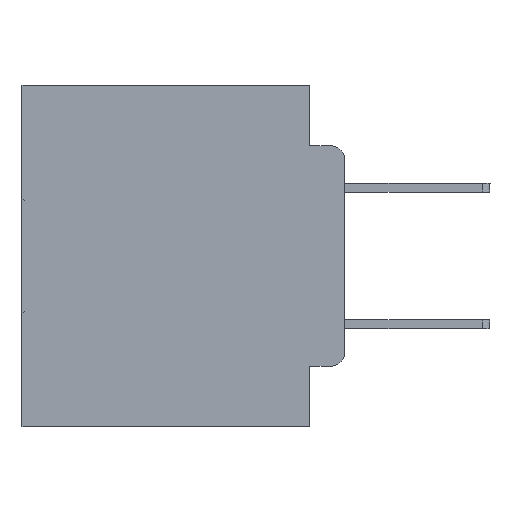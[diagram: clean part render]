
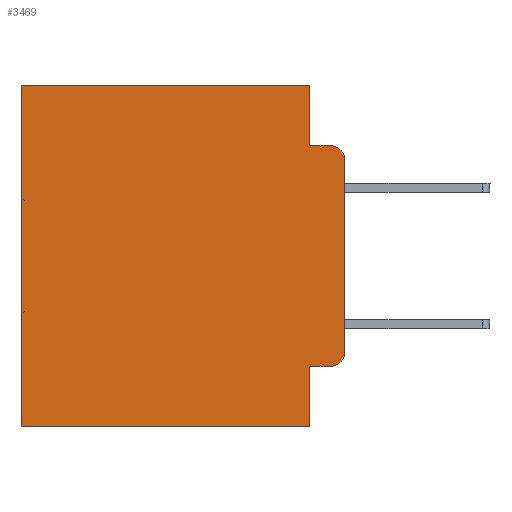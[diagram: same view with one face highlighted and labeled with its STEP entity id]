
A CAD part, left-side view. The second image highlights one B-rep face of the part: STEP entity #3469.
In plain terms, the highlighted planar face has unit normal (-1, 0, 0).
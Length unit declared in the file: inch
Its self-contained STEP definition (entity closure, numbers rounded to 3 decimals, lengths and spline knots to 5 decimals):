
#655 = PLANE ( 'NONE',  #26669 ) ;
#784 = VECTOR ( 'NONE', #4805, 39.37008 ) ;
#868 = ORIENTED_EDGE ( 'NONE', *, *, #27273, .F. ) ;
#1211 = LINE ( 'NONE', #33063, #5243 ) ;
#1711 = VERTEX_POINT ( 'NONE', #8303 ) ;
#1986 = LINE ( 'NONE', #26857, #13638 ) ;
#2028 = FACE_OUTER_BOUND ( 'NONE', #18112, .T. ) ;
#3469 = ADVANCED_FACE ( 'NONE', ( #2028 ), #655, .F. ) ;
#3505 = AXIS2_PLACEMENT_3D ( 'NONE', #26942, #3842, #11564 ) ;
#3672 = DIRECTION ( 'NONE',  ( 0., 0., -1. ) ) ;
#3842 = DIRECTION ( 'NONE',  ( -1., 0., 0. ) ) ;
#4103 = DIRECTION ( 'NONE',  ( 0., 1., 0. ) ) ;
#4350 = EDGE_CURVE ( 'NONE', #14975, #30432, #7971, .T. ) ;
#4805 = DIRECTION ( 'NONE',  ( 0., 0., -1. ) ) ;
#5243 = VECTOR ( 'NONE', #10487, 39.37008 ) ;
#6260 = CARTESIAN_POINT ( 'NONE',  ( 0.298, 0.051, -0.4115 ) ) ;
#6262 = CIRCLE ( 'NONE', #3505, 0.02 ) ;
#7115 = CARTESIAN_POINT ( 'NONE',  ( 0.298, 0.051, -0.4115 ) ) ;
#7971 = LINE ( 'NONE', #18853, #24042 ) ;
#8038 = LINE ( 'NONE', #26009, #16070 ) ;
#8303 = CARTESIAN_POINT ( 'NONE',  ( 0.298, 0.473, 0. ) ) ;
#8519 = LINE ( 'NONE', #32866, #29829 ) ;
#9016 = DIRECTION ( 'NONE',  ( 0., -1., 0. ) ) ;
#9346 = VECTOR ( 'NONE', #21814, 39.37008 ) ;
#10036 = CARTESIAN_POINT ( 'NONE',  ( 0.298, 0.02, -0.4115 ) ) ;
#10487 = DIRECTION ( 'NONE',  ( 0., 1., 0. ) ) ;
#10829 = EDGE_CURVE ( 'NONE', #14975, #21469, #29065, .T. ) ;
#11564 = DIRECTION ( 'NONE',  ( 0., 0., -1. ) ) ;
#12531 = AXIS2_PLACEMENT_3D ( 'NONE', #19474, #24577, #24689 ) ;
#13233 = EDGE_CURVE ( 'NONE', #21469, #29718, #6262, .T. ) ;
#13358 = VECTOR ( 'NONE', #9016, 39.37008 ) ;
#13638 = VECTOR ( 'NONE', #4103, 39.37008 ) ;
#14143 = CARTESIAN_POINT ( 'NONE',  ( 0.298, 0.02, -0.0885 ) ) ;
#14159 = EDGE_CURVE ( 'NONE', #14257, #26178, #31507, .T. ) ;
#14257 = VERTEX_POINT ( 'NONE', #19915 ) ;
#14975 = VERTEX_POINT ( 'NONE', #7115 ) ;
#15673 = EDGE_CURVE ( 'NONE', #14257, #29718, #8519, .T. ) ;
#16070 = VECTOR ( 'NONE', #31281, 39.37008 ) ;
#16221 = CARTESIAN_POINT ( 'NONE',  ( 0.298, 0., 0. ) ) ;
#16956 = DIRECTION ( 'NONE',  ( 0., 0., -1. ) ) ;
#17790 = CARTESIAN_POINT ( 'NONE',  ( 0.298, 0.051, -0.5 ) ) ;
#18037 = EDGE_CURVE ( 'NONE', #1711, #30231, #24470, .T. ) ;
#18072 = ORIENTED_EDGE ( 'NONE', *, *, #4350, .F. ) ;
#18112 = EDGE_LOOP ( 'NONE', ( #28570, #24672, #868, #29289, #29490, #26769, #25719, #18072, #19033, #26570 ) ) ;
#18853 = CARTESIAN_POINT ( 'NONE',  ( 0.298, 0.051, 0. ) ) ;
#19033 = ORIENTED_EDGE ( 'NONE', *, *, #10829, .T. ) ;
#19474 = CARTESIAN_POINT ( 'NONE',  ( 0.298, 0.02, -0.1085 ) ) ;
#19830 = DIRECTION ( 'NONE',  ( 0., 0., -1. ) ) ;
#19915 = CARTESIAN_POINT ( 'NONE',  ( 0.298, 0., -0.1085 ) ) ;
#20411 = CARTESIAN_POINT ( 'NONE',  ( 0.298, 0.051, -0.0885 ) ) ;
#20499 = CARTESIAN_POINT ( 'NONE',  ( 0.298, 0., -0.3915 ) ) ;
#21469 = VERTEX_POINT ( 'NONE', #10036 ) ;
#21702 = VERTEX_POINT ( 'NONE', #27605 ) ;
#21814 = DIRECTION ( 'NONE',  ( 0., -1., 0. ) ) ;
#22662 = VERTEX_POINT ( 'NONE', #20411 ) ;
#23863 = EDGE_CURVE ( 'NONE', #30432, #30231, #1211, .T. ) ;
#24042 = VECTOR ( 'NONE', #16956, 39.37008 ) ;
#24186 = CARTESIAN_POINT ( 'NONE',  ( 0.298, 0.051, -0.0885 ) ) ;
#24239 = EDGE_CURVE ( 'NONE', #21702, #1711, #1986, .T. ) ;
#24470 = LINE ( 'NONE', #27464, #784 ) ;
#24577 = DIRECTION ( 'NONE',  ( -1., 0., 0. ) ) ;
#24672 = ORIENTED_EDGE ( 'NONE', *, *, #14159, .T. ) ;
#24689 = DIRECTION ( 'NONE',  ( 0., 0., -1. ) ) ;
#25405 = LINE ( 'NONE', #24186, #13358 ) ;
#25719 = ORIENTED_EDGE ( 'NONE', *, *, #23863, .F. ) ;
#26009 = CARTESIAN_POINT ( 'NONE',  ( 0.298, 0.051, 0. ) ) ;
#26178 = VERTEX_POINT ( 'NONE', #14143 ) ;
#26570 = ORIENTED_EDGE ( 'NONE', *, *, #13233, .T. ) ;
#26669 = AXIS2_PLACEMENT_3D ( 'NONE', #16221, #29167, #3672 ) ;
#26769 = ORIENTED_EDGE ( 'NONE', *, *, #18037, .T. ) ;
#26857 = CARTESIAN_POINT ( 'NONE',  ( 0.298, 0., 0. ) ) ;
#26942 = CARTESIAN_POINT ( 'NONE',  ( 0.298, 0.02, -0.3915 ) ) ;
#27273 = EDGE_CURVE ( 'NONE', #22662, #26178, #25405, .T. ) ;
#27464 = CARTESIAN_POINT ( 'NONE',  ( 0.298, 0.473, 0. ) ) ;
#27605 = CARTESIAN_POINT ( 'NONE',  ( 0.298, 0.051, 0. ) ) ;
#28570 = ORIENTED_EDGE ( 'NONE', *, *, #15673, .F. ) ;
#29065 = LINE ( 'NONE', #6260, #9346 ) ;
#29167 = DIRECTION ( 'NONE',  ( 1., 0., 0. ) ) ;
#29289 = ORIENTED_EDGE ( 'NONE', *, *, #32543, .F. ) ;
#29490 = ORIENTED_EDGE ( 'NONE', *, *, #24239, .T. ) ;
#29718 = VERTEX_POINT ( 'NONE', #20499 ) ;
#29829 = VECTOR ( 'NONE', #19830, 39.37008 ) ;
#30231 = VERTEX_POINT ( 'NONE', #32956 ) ;
#30432 = VERTEX_POINT ( 'NONE', #17790 ) ;
#31281 = DIRECTION ( 'NONE',  ( 0., 0., -1. ) ) ;
#31507 = CIRCLE ( 'NONE', #12531, 0.02 ) ;
#32543 = EDGE_CURVE ( 'NONE', #21702, #22662, #8038, .T. ) ;
#32866 = CARTESIAN_POINT ( 'NONE',  ( 0.298, 0., 0. ) ) ;
#32956 = CARTESIAN_POINT ( 'NONE',  ( 0.298, 0.473, -0.5 ) ) ;
#33063 = CARTESIAN_POINT ( 'NONE',  ( 0.298, 0., -0.5 ) ) ;
